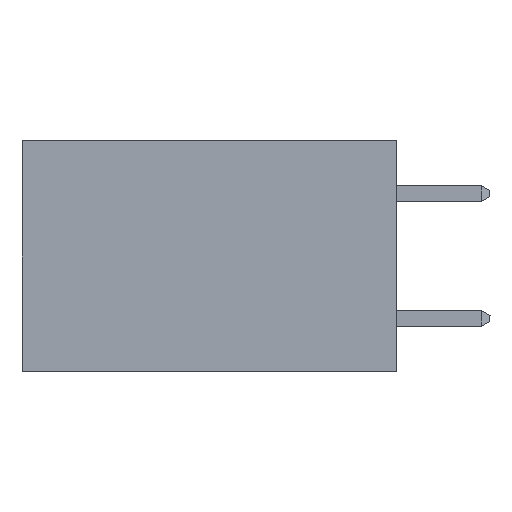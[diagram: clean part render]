
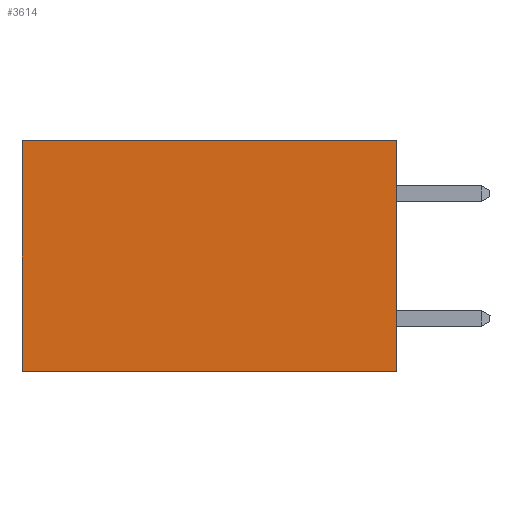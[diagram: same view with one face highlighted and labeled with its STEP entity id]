
A CAD part, left-side view. The second image highlights one B-rep face of the part: STEP entity #3614.
In plain terms, the highlighted planar face has unit normal (-1, 0, 0).
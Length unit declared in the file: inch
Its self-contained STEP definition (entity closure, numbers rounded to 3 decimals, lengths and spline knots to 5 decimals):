
#633 = ORIENTED_EDGE ( 'NONE', *, *, #4680, .T. ) ;
#1355 = LINE ( 'NONE', #8521, #3441 ) ;
#1583 = DIRECTION ( 'NONE',  ( 0., 0., -1. ) ) ;
#1686 = CARTESIAN_POINT ( 'NONE',  ( 0.2615, 0.6, -0.37 ) ) ;
#1932 = CARTESIAN_POINT ( 'NONE',  ( 0.2615, 0., 0. ) ) ;
#1980 = VECTOR ( 'NONE', #2650, 39.37008 ) ;
#1982 = CARTESIAN_POINT ( 'NONE',  ( 0.2615, 0.6, -0.37 ) ) ;
#2092 = ORIENTED_EDGE ( 'NONE', *, *, #3685, .F. ) ;
#2531 = VERTEX_POINT ( 'NONE', #1982 ) ;
#2650 = DIRECTION ( 'NONE',  ( 0., 0., -1. ) ) ;
#2662 = CARTESIAN_POINT ( 'NONE',  ( 0.2615, 0., -0.37 ) ) ;
#3416 = LINE ( 'NONE', #1686, #5527 ) ;
#3441 = VECTOR ( 'NONE', #8573, 39.37008 ) ;
#3499 = VERTEX_POINT ( 'NONE', #10126 ) ;
#3614 = ADVANCED_FACE ( 'NONE', ( #11182 ), #9093, .F. ) ;
#3685 = EDGE_CURVE ( 'NONE', #10032, #2531, #1355, .T. ) ;
#3696 = ORIENTED_EDGE ( 'NONE', *, *, #10894, .T. ) ;
#4394 = LINE ( 'NONE', #10902, #11008 ) ;
#4680 = EDGE_CURVE ( 'NONE', #3499, #2531, #3416, .T. ) ;
#4690 = LINE ( 'NONE', #7967, #1980 ) ;
#5527 = VECTOR ( 'NONE', #1583, 39.37008 ) ;
#7967 = CARTESIAN_POINT ( 'NONE',  ( 0.2615, 0., -0.37 ) ) ;
#8257 = EDGE_LOOP ( 'NONE', ( #633, #2092, #8786, #3696 ) ) ;
#8374 = DIRECTION ( 'NONE',  ( 0., 1., 0. ) ) ;
#8521 = CARTESIAN_POINT ( 'NONE',  ( 0.2615, 0., -0.37 ) ) ;
#8573 = DIRECTION ( 'NONE',  ( 0., 1., 0. ) ) ;
#8786 = ORIENTED_EDGE ( 'NONE', *, *, #10616, .F. ) ;
#8883 = AXIS2_PLACEMENT_3D ( 'NONE', #9004, #8990, #8967 ) ;
#8967 = DIRECTION ( 'NONE',  ( 0., 0., -1. ) ) ;
#8990 = DIRECTION ( 'NONE',  ( 1., 0., 0. ) ) ;
#9004 = CARTESIAN_POINT ( 'NONE',  ( 0.2615, 0., -0.37 ) ) ;
#9093 = PLANE ( 'NONE',  #8883 ) ;
#9289 = VERTEX_POINT ( 'NONE', #1932 ) ;
#10032 = VERTEX_POINT ( 'NONE', #2662 ) ;
#10126 = CARTESIAN_POINT ( 'NONE',  ( 0.2615, 0.6, 0. ) ) ;
#10616 = EDGE_CURVE ( 'NONE', #9289, #10032, #4690, .T. ) ;
#10894 = EDGE_CURVE ( 'NONE', #9289, #3499, #4394, .T. ) ;
#10902 = CARTESIAN_POINT ( 'NONE',  ( 0.2615, 0., 0. ) ) ;
#11008 = VECTOR ( 'NONE', #8374, 39.37008 ) ;
#11182 = FACE_OUTER_BOUND ( 'NONE', #8257, .T. ) ;
